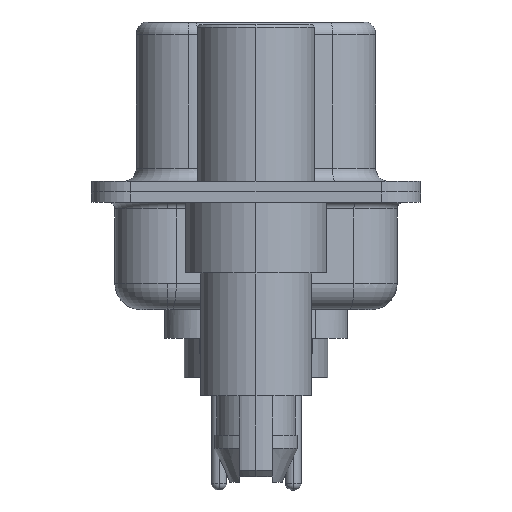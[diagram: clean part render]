
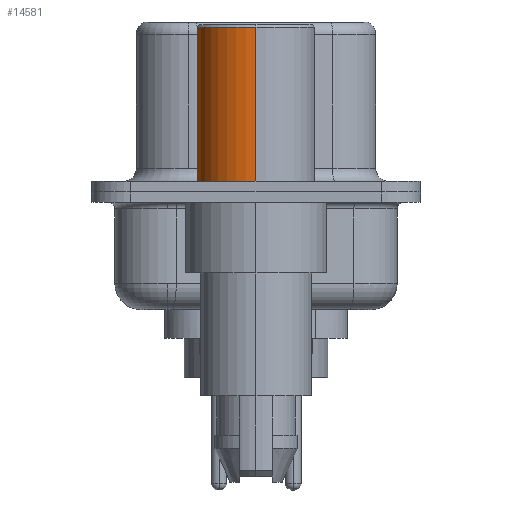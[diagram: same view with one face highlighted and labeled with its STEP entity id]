
A CAD part, left-side view. The second image highlights one B-rep face of the part: STEP entity #14581.
In plain terms, the highlighted cylindrical face has radius 2.25 mm (diameter 4.5 mm), a partial arc.
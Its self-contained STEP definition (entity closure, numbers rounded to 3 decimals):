
#58 = LINE ( 'NONE', #14790, #10777 ) ;
#120 = EDGE_LOOP ( 'NONE', ( #17136, #16387, #15866, #16039 ) ) ;
#697 = VERTEX_POINT ( 'NONE', #15222 ) ;
#765 = AXIS2_PLACEMENT_3D ( 'NONE', #9649, #1668, #11070 ) ;
#1187 = LINE ( 'NONE', #5892, #7395 ) ;
#1234 = CARTESIAN_POINT ( 'NONE',  ( 2.25, 0., 0.4 ) ) ;
#1668 = DIRECTION ( 'NONE',  ( 0., 0., 1. ) ) ;
#1806 = AXIS2_PLACEMENT_3D ( 'NONE', #1926, #7258, #9974 ) ;
#1926 = CARTESIAN_POINT ( 'NONE',  ( 0., 0., 0.581 ) ) ;
#2826 = CYLINDRICAL_SURFACE ( 'NONE', #1806, 2.25 ) ;
#3092 = AXIS2_PLACEMENT_3D ( 'NONE', #10857, #5756, #12257 ) ;
#3871 = EDGE_CURVE ( 'NONE', #697, #15706, #16383, .T. ) ;
#4317 = CIRCLE ( 'NONE', #765, 2.25 ) ;
#4513 = CARTESIAN_POINT ( 'NONE',  ( -2.25, 0., 0.4 ) ) ;
#5224 = DIRECTION ( 'NONE',  ( 0., 0., 1. ) ) ;
#5690 = EDGE_CURVE ( 'NONE', #9743, #15706, #1187, .T. ) ;
#5756 = DIRECTION ( 'NONE',  ( 0., 0., 1. ) ) ;
#5892 = CARTESIAN_POINT ( 'NONE',  ( -2.25, 0., 0.581 ) ) ;
#7258 = DIRECTION ( 'NONE',  ( 0., 0., 1. ) ) ;
#7395 = VECTOR ( 'NONE', #16855, 1000. ) ;
#9649 = CARTESIAN_POINT ( 'NONE',  ( 0., 0., 0.4 ) ) ;
#9743 = VERTEX_POINT ( 'NONE', #4513 ) ;
#9974 = DIRECTION ( 'NONE',  ( 1., 0., 0. ) ) ;
#10777 = VECTOR ( 'NONE', #5224, 1000. ) ;
#10857 = CARTESIAN_POINT ( 'NONE',  ( 0., 0., 6.3 ) ) ;
#11070 = DIRECTION ( 'NONE',  ( 1., 0., 0. ) ) ;
#11854 = EDGE_CURVE ( 'NONE', #16491, #9743, #4317, .T. ) ;
#12257 = DIRECTION ( 'NONE',  ( 1., 0., 0. ) ) ;
#13687 = FACE_OUTER_BOUND ( 'NONE', #120, .T. ) ;
#14581 = ADVANCED_FACE ( 'NONE', ( #13687 ), #2826, .T. ) ;
#14790 = CARTESIAN_POINT ( 'NONE',  ( 2.25, 0., 0.581 ) ) ;
#15026 = CARTESIAN_POINT ( 'NONE',  ( -2.25, 0., 6.3 ) ) ;
#15222 = CARTESIAN_POINT ( 'NONE',  ( 2.25, 0., 6.3 ) ) ;
#15706 = VERTEX_POINT ( 'NONE', #15026 ) ;
#15866 = ORIENTED_EDGE ( 'NONE', *, *, #3871, .F. ) ;
#16039 = ORIENTED_EDGE ( 'NONE', *, *, #16291, .F. ) ;
#16291 = EDGE_CURVE ( 'NONE', #16491, #697, #58, .T. ) ;
#16383 = CIRCLE ( 'NONE', #3092, 2.25 ) ;
#16387 = ORIENTED_EDGE ( 'NONE', *, *, #5690, .T. ) ;
#16491 = VERTEX_POINT ( 'NONE', #1234 ) ;
#16855 = DIRECTION ( 'NONE',  ( 0., 0., 1. ) ) ;
#17136 = ORIENTED_EDGE ( 'NONE', *, *, #11854, .T. ) ;
